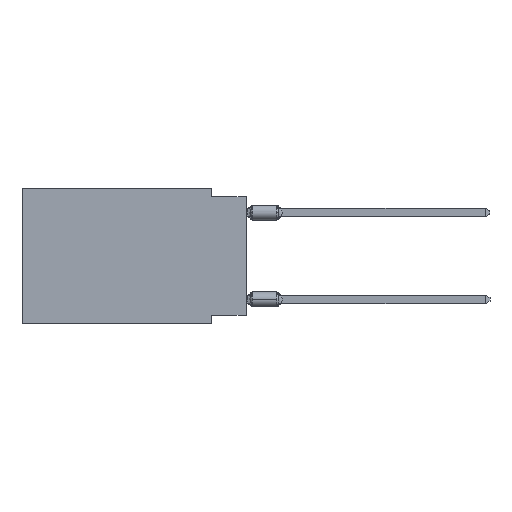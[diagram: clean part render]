
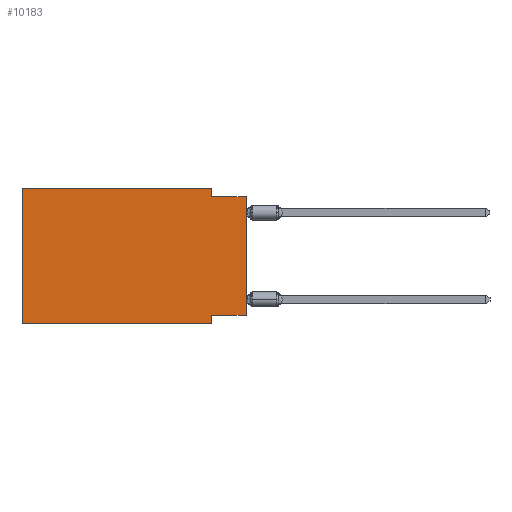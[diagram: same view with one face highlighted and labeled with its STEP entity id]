
A CAD part, left-side view. The second image highlights one B-rep face of the part: STEP entity #10183.
In plain terms, the highlighted planar face has unit normal (-1, 0, 0).
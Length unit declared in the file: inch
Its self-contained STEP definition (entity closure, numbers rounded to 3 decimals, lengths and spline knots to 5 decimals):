
#50 = CARTESIAN_POINT ( 'NONE',  ( 0., 0., -0.025 ) ) ;
#286 = CARTESIAN_POINT ( 'NONE',  ( 0., 0.645, 0. ) ) ;
#1212 = LINE ( 'NONE', #12949, #12895 ) ;
#1476 = CARTESIAN_POINT ( 'NONE',  ( 0., 0.1, -0.365 ) ) ;
#1550 = DIRECTION ( 'NONE',  ( 0., 0., -1. ) ) ;
#1577 = DIRECTION ( 'NONE',  ( 0., -1., 0. ) ) ;
#2779 = EDGE_CURVE ( 'NONE', #5732, #14916, #25982, .T. ) ;
#3010 = VECTOR ( 'NONE', #1577, 39.37008 ) ;
#3090 = DIRECTION ( 'NONE',  ( 0., 0., -1. ) ) ;
#3109 = ORIENTED_EDGE ( 'NONE', *, *, #8041, .F. ) ;
#3407 = DIRECTION ( 'NONE',  ( 1., 0., 0. ) ) ;
#3579 = ORIENTED_EDGE ( 'NONE', *, *, #2779, .F. ) ;
#3859 = VERTEX_POINT ( 'NONE', #10059 ) ;
#3872 = VECTOR ( 'NONE', #1550, 39.37008 ) ;
#4069 = DIRECTION ( 'NONE',  ( 0., 1., 0. ) ) ;
#5642 = LINE ( 'NONE', #19639, #3872 ) ;
#5732 = VERTEX_POINT ( 'NONE', #27615 ) ;
#5958 = LINE ( 'NONE', #8221, #3010 ) ;
#6378 = CARTESIAN_POINT ( 'NONE',  ( 0., 0., 0. ) ) ;
#6436 = VERTEX_POINT ( 'NONE', #11523 ) ;
#7346 = EDGE_CURVE ( 'NONE', #14916, #29531, #27913, .T. ) ;
#7832 = DIRECTION ( 'NONE',  ( 0., 0., 1. ) ) ;
#8040 = VERTEX_POINT ( 'NONE', #17482 ) ;
#8041 = EDGE_CURVE ( 'NONE', #3859, #14281, #1212, .T. ) ;
#8221 = CARTESIAN_POINT ( 'NONE',  ( 0., 0.645, -0.39 ) ) ;
#9441 = ORIENTED_EDGE ( 'NONE', *, *, #10589, .F. ) ;
#10059 = CARTESIAN_POINT ( 'NONE',  ( 0., 0., -0.365 ) ) ;
#10183 = ADVANCED_FACE ( 'NONE', ( #10484 ), #26885, .F. ) ;
#10484 = FACE_OUTER_BOUND ( 'NONE', #28815, .T. ) ;
#10589 = EDGE_CURVE ( 'NONE', #14281, #6436, #5642, .T. ) ;
#11442 = VECTOR ( 'NONE', #7832, 39.37008 ) ;
#11523 = CARTESIAN_POINT ( 'NONE',  ( 0., 0.1, -0.39 ) ) ;
#12895 = VECTOR ( 'NONE', #4069, 39.37008 ) ;
#12927 = CARTESIAN_POINT ( 'NONE',  ( 0., 0.645, 0. ) ) ;
#12949 = CARTESIAN_POINT ( 'NONE',  ( 0., 0., -0.365 ) ) ;
#13456 = VECTOR ( 'NONE', #18883, 39.37008 ) ;
#13999 = EDGE_CURVE ( 'NONE', #3859, #29531, #22619, .T. ) ;
#14281 = VERTEX_POINT ( 'NONE', #1476 ) ;
#14435 = AXIS2_PLACEMENT_3D ( 'NONE', #28724, #3407, #15154 ) ;
#14916 = VERTEX_POINT ( 'NONE', #25138 ) ;
#15154 = DIRECTION ( 'NONE',  ( 0., 0., -1. ) ) ;
#15379 = CARTESIAN_POINT ( 'NONE',  ( 0., 0., -0.025 ) ) ;
#16161 = EDGE_CURVE ( 'NONE', #18486, #5732, #24844, .T. ) ;
#16940 = CARTESIAN_POINT ( 'NONE',  ( 0., 0.645, 0. ) ) ;
#17482 = CARTESIAN_POINT ( 'NONE',  ( 0., 0.645, -0.39 ) ) ;
#17819 = DIRECTION ( 'NONE',  ( 0., 0., 1. ) ) ;
#17869 = VECTOR ( 'NONE', #3090, 39.37008 ) ;
#18486 = VERTEX_POINT ( 'NONE', #16940 ) ;
#18883 = DIRECTION ( 'NONE',  ( 0., -1., 0. ) ) ;
#19639 = CARTESIAN_POINT ( 'NONE',  ( 0., 0.1, -0.39 ) ) ;
#20758 = ORIENTED_EDGE ( 'NONE', *, *, #27451, .T. ) ;
#20809 = EDGE_CURVE ( 'NONE', #8040, #18486, #24379, .T. ) ;
#21398 = VECTOR ( 'NONE', #24987, 39.37008 ) ;
#22619 = LINE ( 'NONE', #6378, #26536 ) ;
#23719 = CARTESIAN_POINT ( 'NONE',  ( 0., 0.1, 0. ) ) ;
#24379 = LINE ( 'NONE', #12927, #11442 ) ;
#24844 = LINE ( 'NONE', #286, #21398 ) ;
#24987 = DIRECTION ( 'NONE',  ( 0., -1., 0. ) ) ;
#25138 = CARTESIAN_POINT ( 'NONE',  ( 0., 0.1, -0.025 ) ) ;
#25267 = ORIENTED_EDGE ( 'NONE', *, *, #20809, .F. ) ;
#25835 = ORIENTED_EDGE ( 'NONE', *, *, #16161, .F. ) ;
#25844 = ORIENTED_EDGE ( 'NONE', *, *, #13999, .T. ) ;
#25982 = LINE ( 'NONE', #23719, #17869 ) ;
#26022 = ORIENTED_EDGE ( 'NONE', *, *, #7346, .F. ) ;
#26536 = VECTOR ( 'NONE', #17819, 39.37008 ) ;
#26885 = PLANE ( 'NONE',  #14435 ) ;
#27451 = EDGE_CURVE ( 'NONE', #8040, #6436, #5958, .T. ) ;
#27615 = CARTESIAN_POINT ( 'NONE',  ( 0., 0.1, 0. ) ) ;
#27913 = LINE ( 'NONE', #50, #13456 ) ;
#28724 = CARTESIAN_POINT ( 'NONE',  ( 0., 0.645, 0. ) ) ;
#28815 = EDGE_LOOP ( 'NONE', ( #25844, #26022, #3579, #25835, #25267, #20758, #9441, #3109 ) ) ;
#29531 = VERTEX_POINT ( 'NONE', #15379 ) ;
